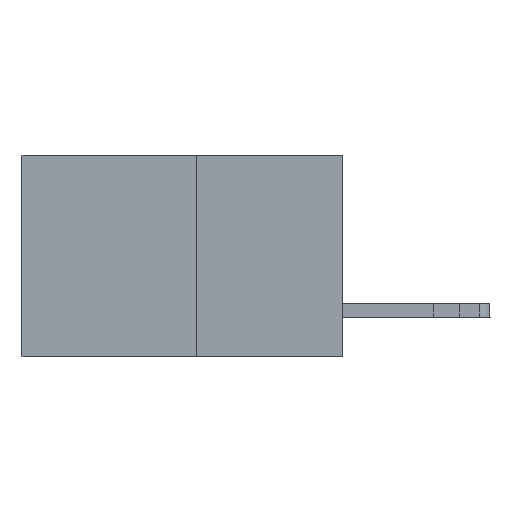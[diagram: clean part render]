
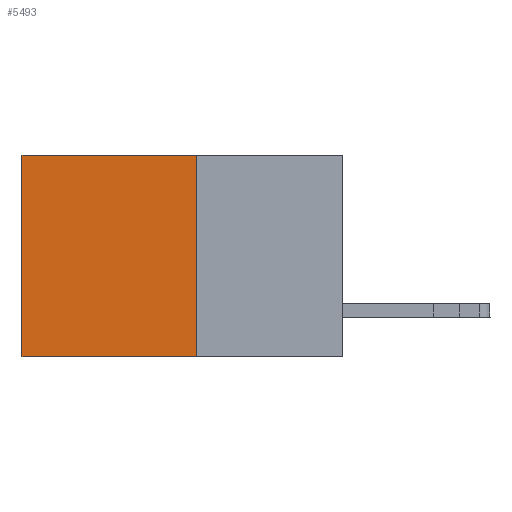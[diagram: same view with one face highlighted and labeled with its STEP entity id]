
A CAD part, left-side view. The second image highlights one B-rep face of the part: STEP entity #5493.
In plain terms, the highlighted planar face has unit normal (-1, 0, 0).
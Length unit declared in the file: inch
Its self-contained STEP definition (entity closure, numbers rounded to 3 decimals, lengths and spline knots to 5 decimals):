
#320 = CARTESIAN_POINT ( 'NONE',  ( 0.277, 0.27, -0.37 ) ) ;
#330 = DIRECTION ( 'NONE',  ( 0., 0., -1. ) ) ;
#548 = LINE ( 'NONE', #11847, #8697 ) ;
#1507 = LINE ( 'NONE', #22102, #17883 ) ;
#1514 = DIRECTION ( 'NONE',  ( 1., 0., 0. ) ) ;
#2720 = EDGE_CURVE ( 'NONE', #12639, #4668, #6265, .T. ) ;
#4668 = VERTEX_POINT ( 'NONE', #14885 ) ;
#5354 = DIRECTION ( 'NONE',  ( 0., 0., -1. ) ) ;
#5370 = AXIS2_PLACEMENT_3D ( 'NONE', #15038, #1514, #13195 ) ;
#5493 = ADVANCED_FACE ( 'NONE', ( #12814 ), #13061, .F. ) ;
#6265 = LINE ( 'NONE', #15460, #16301 ) ;
#8697 = VECTOR ( 'NONE', #15679, 39.37008 ) ;
#8952 = EDGE_CURVE ( 'NONE', #18692, #12639, #548, .T. ) ;
#9630 = LINE ( 'NONE', #320, #11524 ) ;
#9990 = DIRECTION ( 'NONE',  ( 0., 1., 0. ) ) ;
#10507 = ORIENTED_EDGE ( 'NONE', *, *, #8952, .T. ) ;
#10873 = ORIENTED_EDGE ( 'NONE', *, *, #2720, .T. ) ;
#11178 = CARTESIAN_POINT ( 'NONE',  ( 0.277, 0.59, 0. ) ) ;
#11524 = VECTOR ( 'NONE', #9990, 39.37008 ) ;
#11847 = CARTESIAN_POINT ( 'NONE',  ( 0.277, 0.27, 0. ) ) ;
#12639 = VERTEX_POINT ( 'NONE', #11178 ) ;
#12814 = FACE_OUTER_BOUND ( 'NONE', #15180, .T. ) ;
#13061 = PLANE ( 'NONE',  #5370 ) ;
#13147 = VERTEX_POINT ( 'NONE', #19549 ) ;
#13195 = DIRECTION ( 'NONE',  ( 0., 0., -1. ) ) ;
#14885 = CARTESIAN_POINT ( 'NONE',  ( 0.277, 0.59, -0.37 ) ) ;
#15038 = CARTESIAN_POINT ( 'NONE',  ( 0.277, 0.27, -0.37 ) ) ;
#15180 = EDGE_LOOP ( 'NONE', ( #10873, #24282, #21794, #10507 ) ) ;
#15460 = CARTESIAN_POINT ( 'NONE',  ( 0.277, 0.59, -0.37 ) ) ;
#15656 = EDGE_CURVE ( 'NONE', #13147, #4668, #9630, .T. ) ;
#15679 = DIRECTION ( 'NONE',  ( 0., 1., 0. ) ) ;
#16301 = VECTOR ( 'NONE', #330, 39.37008 ) ;
#16457 = EDGE_CURVE ( 'NONE', #18692, #13147, #1507, .T. ) ;
#17883 = VECTOR ( 'NONE', #5354, 39.37008 ) ;
#18692 = VERTEX_POINT ( 'NONE', #21844 ) ;
#19549 = CARTESIAN_POINT ( 'NONE',  ( 0.277, 0.27, -0.37 ) ) ;
#21794 = ORIENTED_EDGE ( 'NONE', *, *, #16457, .F. ) ;
#21844 = CARTESIAN_POINT ( 'NONE',  ( 0.277, 0.27, 0. ) ) ;
#22102 = CARTESIAN_POINT ( 'NONE',  ( 0.277, 0.27, -0.37 ) ) ;
#24282 = ORIENTED_EDGE ( 'NONE', *, *, #15656, .F. ) ;
